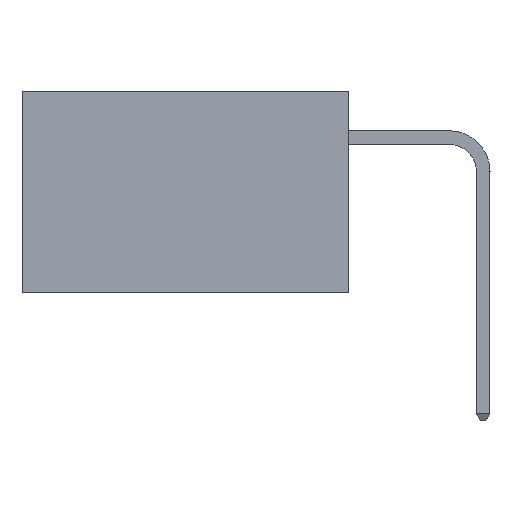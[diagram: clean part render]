
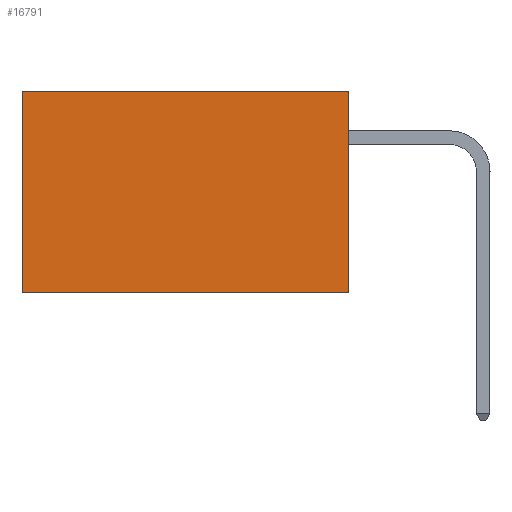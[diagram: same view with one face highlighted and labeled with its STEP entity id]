
A CAD part, left-side view. The second image highlights one B-rep face of the part: STEP entity #16791.
In plain terms, the highlighted planar face has unit normal (-1, 0, 0).
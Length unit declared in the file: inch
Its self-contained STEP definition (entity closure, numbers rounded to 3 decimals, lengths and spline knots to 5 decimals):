
#323 = ORIENTED_EDGE ( 'NONE', *, *, #22234, .F. ) ;
#392 = LINE ( 'NONE', #28797, #11592 ) ;
#519 = ORIENTED_EDGE ( 'NONE', *, *, #22314, .T. ) ;
#1069 = VERTEX_POINT ( 'NONE', #1800 ) ;
#1800 = CARTESIAN_POINT ( 'NONE',  ( 0.2875, 0.6, -0.37 ) ) ;
#2473 = VECTOR ( 'NONE', #10617, 39.37008 ) ;
#2932 = VECTOR ( 'NONE', #18544, 39.37008 ) ;
#4925 = CARTESIAN_POINT ( 'NONE',  ( 0.2875, 0., 0. ) ) ;
#5457 = PLANE ( 'NONE',  #19412 ) ;
#5470 = LINE ( 'NONE', #9789, #11458 ) ;
#6730 = EDGE_CURVE ( 'NONE', #17899, #23566, #5470, .T. ) ;
#7679 = LINE ( 'NONE', #26324, #2473 ) ;
#9789 = CARTESIAN_POINT ( 'NONE',  ( 0.2875, 0., 0. ) ) ;
#9948 = DIRECTION ( 'NONE',  ( 1., 0., 0. ) ) ;
#10617 = DIRECTION ( 'NONE',  ( 0., 1., 0. ) ) ;
#11458 = VECTOR ( 'NONE', #27655, 39.37008 ) ;
#11592 = VECTOR ( 'NONE', #13228, 39.37008 ) ;
#13228 = DIRECTION ( 'NONE',  ( 0., 0., -1. ) ) ;
#13900 = CARTESIAN_POINT ( 'NONE',  ( 0.2875, 0., 0. ) ) ;
#15504 = EDGE_CURVE ( 'NONE', #17899, #15800, #20246, .T. ) ;
#15800 = VERTEX_POINT ( 'NONE', #19500 ) ;
#16329 = FACE_OUTER_BOUND ( 'NONE', #28227, .T. ) ;
#16520 = ORIENTED_EDGE ( 'NONE', *, *, #15504, .F. ) ;
#16791 = ADVANCED_FACE ( 'NONE', ( #16329 ), #5457, .F. ) ;
#17899 = VERTEX_POINT ( 'NONE', #13900 ) ;
#18544 = DIRECTION ( 'NONE',  ( 0., 0., -1. ) ) ;
#19412 = AXIS2_PLACEMENT_3D ( 'NONE', #23365, #9948, #25694 ) ;
#19500 = CARTESIAN_POINT ( 'NONE',  ( 0.2875, 0., -0.37 ) ) ;
#20246 = LINE ( 'NONE', #4925, #2932 ) ;
#22234 = EDGE_CURVE ( 'NONE', #15800, #1069, #7679, .T. ) ;
#22314 = EDGE_CURVE ( 'NONE', #23566, #1069, #392, .T. ) ;
#22821 = ORIENTED_EDGE ( 'NONE', *, *, #6730, .T. ) ;
#23365 = CARTESIAN_POINT ( 'NONE',  ( 0.2875, 0., 0. ) ) ;
#23566 = VERTEX_POINT ( 'NONE', #28833 ) ;
#25694 = DIRECTION ( 'NONE',  ( 0., 0., -1. ) ) ;
#26324 = CARTESIAN_POINT ( 'NONE',  ( 0.2875, 0., -0.37 ) ) ;
#27655 = DIRECTION ( 'NONE',  ( 0., 1., 0. ) ) ;
#28227 = EDGE_LOOP ( 'NONE', ( #519, #323, #16520, #22821 ) ) ;
#28797 = CARTESIAN_POINT ( 'NONE',  ( 0.2875, 0.6, 0. ) ) ;
#28833 = CARTESIAN_POINT ( 'NONE',  ( 0.2875, 0.6, 0. ) ) ;
